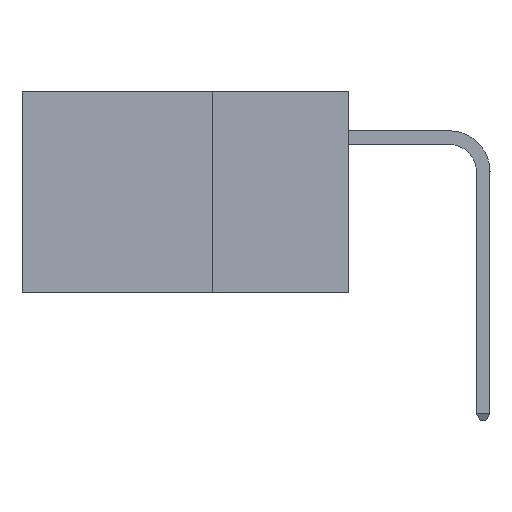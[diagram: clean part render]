
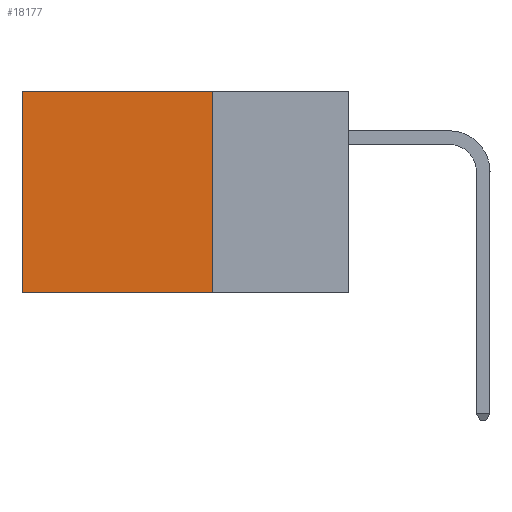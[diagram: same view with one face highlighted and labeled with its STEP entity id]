
A CAD part, left-side view. The second image highlights one B-rep face of the part: STEP entity #18177.
In plain terms, the highlighted planar face has unit normal (-1, 0, 0).
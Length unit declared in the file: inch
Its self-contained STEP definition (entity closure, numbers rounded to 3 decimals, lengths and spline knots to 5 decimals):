
#1881 = ORIENTED_EDGE ( 'NONE', *, *, #29596, .F. ) ;
#2250 = EDGE_CURVE ( 'NONE', #43107, #41689, #17082, .T. ) ;
#3469 = DIRECTION ( 'NONE',  ( 0., 1., 0. ) ) ;
#4141 = VECTOR ( 'NONE', #3469, 39.37008 ) ;
#4239 = VERTEX_POINT ( 'NONE', #20438 ) ;
#12128 = ORIENTED_EDGE ( 'NONE', *, *, #24690, .F. ) ;
#14010 = ORIENTED_EDGE ( 'NONE', *, *, #2250, .T. ) ;
#14210 = DIRECTION ( 'NONE',  ( 0., 1., 0. ) ) ;
#16139 = CARTESIAN_POINT ( 'NONE',  ( 0.2875, 0.25, 0. ) ) ;
#17082 = LINE ( 'NONE', #31999, #44576 ) ;
#18177 = ADVANCED_FACE ( 'NONE', ( #45190 ), #41673, .F. ) ;
#20438 = CARTESIAN_POINT ( 'NONE',  ( 0.2875, 0.25, -0.37 ) ) ;
#20594 = LINE ( 'NONE', #38877, #4141 ) ;
#22347 = EDGE_CURVE ( 'NONE', #35725, #43107, #32018, .T. ) ;
#24690 = EDGE_CURVE ( 'NONE', #4239, #41689, #20594, .T. ) ;
#29111 = CARTESIAN_POINT ( 'NONE',  ( 0.2875, 0.6, -0.37 ) ) ;
#29596 = EDGE_CURVE ( 'NONE', #35725, #4239, #39236, .T. ) ;
#30650 = DIRECTION ( 'NONE',  ( 0., 0., -1. ) ) ;
#31999 = CARTESIAN_POINT ( 'NONE',  ( 0.2875, 0.6, 0. ) ) ;
#32018 = LINE ( 'NONE', #46322, #36981 ) ;
#33104 = ORIENTED_EDGE ( 'NONE', *, *, #22347, .T. ) ;
#35465 = EDGE_LOOP ( 'NONE', ( #14010, #12128, #1881, #33104 ) ) ;
#35725 = VERTEX_POINT ( 'NONE', #37595 ) ;
#35934 = CARTESIAN_POINT ( 'NONE',  ( 0.2875, 0.25, 0. ) ) ;
#36301 = VECTOR ( 'NONE', #39935, 39.37008 ) ;
#36827 = CARTESIAN_POINT ( 'NONE',  ( 0.2875, 0.6, 0. ) ) ;
#36981 = VECTOR ( 'NONE', #14210, 39.37008 ) ;
#37565 = AXIS2_PLACEMENT_3D ( 'NONE', #16139, #44724, #30650 ) ;
#37595 = CARTESIAN_POINT ( 'NONE',  ( 0.2875, 0.25, 0. ) ) ;
#38877 = CARTESIAN_POINT ( 'NONE',  ( 0.2875, 0.25, -0.37 ) ) ;
#39236 = LINE ( 'NONE', #35934, #36301 ) ;
#39738 = DIRECTION ( 'NONE',  ( 0., 0., -1. ) ) ;
#39935 = DIRECTION ( 'NONE',  ( 0., 0., -1. ) ) ;
#41673 = PLANE ( 'NONE',  #37565 ) ;
#41689 = VERTEX_POINT ( 'NONE', #29111 ) ;
#43107 = VERTEX_POINT ( 'NONE', #36827 ) ;
#44576 = VECTOR ( 'NONE', #39738, 39.37008 ) ;
#44724 = DIRECTION ( 'NONE',  ( 1., 0., 0. ) ) ;
#45190 = FACE_OUTER_BOUND ( 'NONE', #35465, .T. ) ;
#46322 = CARTESIAN_POINT ( 'NONE',  ( 0.2875, 0.25, 0. ) ) ;
